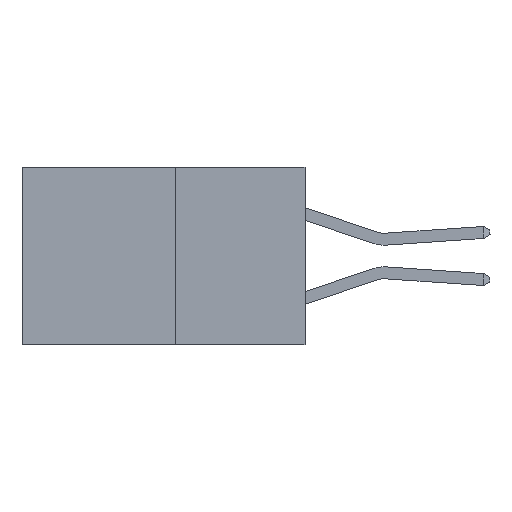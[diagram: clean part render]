
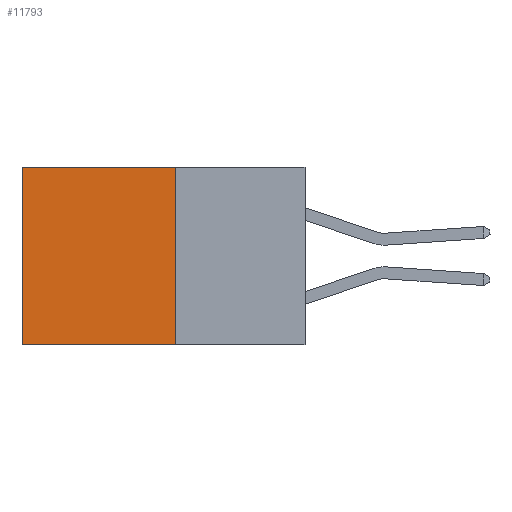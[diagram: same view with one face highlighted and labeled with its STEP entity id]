
A CAD part, left-side view. The second image highlights one B-rep face of the part: STEP entity #11793.
In plain terms, the highlighted planar face has unit normal (-1, 0, 0).
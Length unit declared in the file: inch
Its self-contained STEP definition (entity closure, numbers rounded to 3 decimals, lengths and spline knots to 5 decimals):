
#257 = VECTOR ( 'NONE', #6108, 39.37008 ) ;
#345 = LINE ( 'NONE', #1993, #12223 ) ;
#997 = DIRECTION ( 'NONE',  ( 0., 0., -1. ) ) ;
#1098 = EDGE_CURVE ( 'NONE', #1522, #10259, #7169, .T. ) ;
#1522 = VERTEX_POINT ( 'NONE', #12139 ) ;
#1683 = DIRECTION ( 'NONE',  ( 0., 1., 0. ) ) ;
#1993 = CARTESIAN_POINT ( 'NONE',  ( 0.277, 0.27, -0.37 ) ) ;
#2275 = PLANE ( 'NONE',  #12472 ) ;
#2382 = CARTESIAN_POINT ( 'NONE',  ( 0.277, 0.59, 0. ) ) ;
#3461 = DIRECTION ( 'NONE',  ( 1., 0., 0. ) ) ;
#5631 = FACE_OUTER_BOUND ( 'NONE', #14631, .T. ) ;
#6108 = DIRECTION ( 'NONE',  ( 0., 1., 0. ) ) ;
#6696 = CARTESIAN_POINT ( 'NONE',  ( 0.277, 0.27, -0.37 ) ) ;
#6719 = CARTESIAN_POINT ( 'NONE',  ( 0.277, 0.59, -0.37 ) ) ;
#6810 = LINE ( 'NONE', #13496, #9508 ) ;
#7005 = ORIENTED_EDGE ( 'NONE', *, *, #14786, .T. ) ;
#7147 = ORIENTED_EDGE ( 'NONE', *, *, #1098, .F. ) ;
#7169 = LINE ( 'NONE', #6696, #257 ) ;
#7369 = CARTESIAN_POINT ( 'NONE',  ( 0.277, 0.27, 0. ) ) ;
#7880 = ORIENTED_EDGE ( 'NONE', *, *, #10136, .F. ) ;
#8306 = ORIENTED_EDGE ( 'NONE', *, *, #12062, .T. ) ;
#8841 = VECTOR ( 'NONE', #1683, 39.37008 ) ;
#9039 = CARTESIAN_POINT ( 'NONE',  ( 0.277, 0.27, -0.37 ) ) ;
#9508 = VECTOR ( 'NONE', #997, 39.37008 ) ;
#9579 = VERTEX_POINT ( 'NONE', #2382 ) ;
#10136 = EDGE_CURVE ( 'NONE', #12932, #1522, #345, .T. ) ;
#10259 = VERTEX_POINT ( 'NONE', #6719 ) ;
#11120 = DIRECTION ( 'NONE',  ( 0., 0., -1. ) ) ;
#11332 = DIRECTION ( 'NONE',  ( 0., 0., -1. ) ) ;
#11793 = ADVANCED_FACE ( 'NONE', ( #5631 ), #2275, .F. ) ;
#11862 = LINE ( 'NONE', #7369, #8841 ) ;
#12062 = EDGE_CURVE ( 'NONE', #12932, #9579, #11862, .T. ) ;
#12139 = CARTESIAN_POINT ( 'NONE',  ( 0.277, 0.27, -0.37 ) ) ;
#12223 = VECTOR ( 'NONE', #11120, 39.37008 ) ;
#12472 = AXIS2_PLACEMENT_3D ( 'NONE', #9039, #3461, #11332 ) ;
#12932 = VERTEX_POINT ( 'NONE', #14044 ) ;
#13496 = CARTESIAN_POINT ( 'NONE',  ( 0.277, 0.59, -0.37 ) ) ;
#14044 = CARTESIAN_POINT ( 'NONE',  ( 0.277, 0.27, 0. ) ) ;
#14631 = EDGE_LOOP ( 'NONE', ( #7005, #7147, #7880, #8306 ) ) ;
#14786 = EDGE_CURVE ( 'NONE', #9579, #10259, #6810, .T. ) ;
